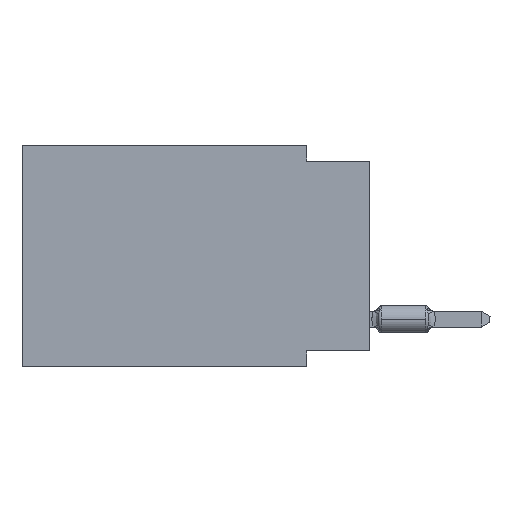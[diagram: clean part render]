
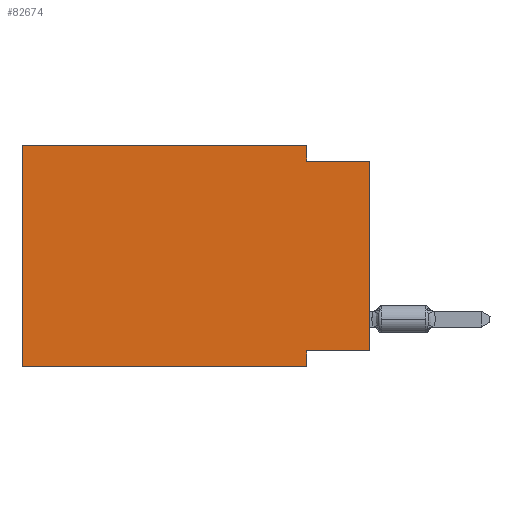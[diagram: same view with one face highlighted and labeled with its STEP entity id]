
A CAD part, left-side view. The second image highlights one B-rep face of the part: STEP entity #82674.
In plain terms, the highlighted planar face has unit normal (-1, 0, 0).
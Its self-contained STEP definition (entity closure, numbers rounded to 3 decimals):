
#1590 = CARTESIAN_POINT ( 'NONE',  ( 0., 0., 0. ) ) ;
#4566 = VECTOR ( 'NONE', #47866, 1000. ) ;
#7027 = VECTOR ( 'NONE', #30321, 1000. ) ;
#7937 = CARTESIAN_POINT ( 'NONE',  ( 0., 13.97, 0. ) ) ;
#10151 = VECTOR ( 'NONE', #42380, 1000. ) ;
#12165 = VERTEX_POINT ( 'NONE', #28537 ) ;
#12567 = ORIENTED_EDGE ( 'NONE', *, *, #30296, .F. ) ;
#13518 = CARTESIAN_POINT ( 'NONE',  ( 0., 0., -8.255 ) ) ;
#17027 = LINE ( 'NONE', #49038, #84397 ) ;
#19657 = ORIENTED_EDGE ( 'NONE', *, *, #29262, .T. ) ;
#20158 = ORIENTED_EDGE ( 'NONE', *, *, #67251, .F. ) ;
#21334 = LINE ( 'NONE', #104791, #4566 ) ;
#22619 = DIRECTION ( 'NONE',  ( 0., 0., -1. ) ) ;
#24917 = LINE ( 'NONE', #1590, #84020 ) ;
#27387 = VECTOR ( 'NONE', #83274, 1000. ) ;
#28537 = CARTESIAN_POINT ( 'NONE',  ( 0., 2.54, -8.255 ) ) ;
#29262 = EDGE_CURVE ( 'NONE', #103199, #61227, #24917, .T. ) ;
#29929 = EDGE_CURVE ( 'NONE', #106783, #54262, #37725, .T. ) ;
#30296 = EDGE_CURVE ( 'NONE', #78901, #106783, #21334, .T. ) ;
#30321 = DIRECTION ( 'NONE',  ( 0., 1., 0. ) ) ;
#30520 = VERTEX_POINT ( 'NONE', #58142 ) ;
#30572 = CARTESIAN_POINT ( 'NONE',  ( 0., 13.97, 0. ) ) ;
#37725 = LINE ( 'NONE', #47454, #77249 ) ;
#38580 = AXIS2_PLACEMENT_3D ( 'NONE', #7937, #41013, #107128 ) ;
#38893 = LINE ( 'NONE', #48086, #71156 ) ;
#41013 = DIRECTION ( 'NONE',  ( 1., 0., 0. ) ) ;
#42380 = DIRECTION ( 'NONE',  ( 0., 0., -1. ) ) ;
#43558 = CARTESIAN_POINT ( 'NONE',  ( 0., 0., -0.635 ) ) ;
#46157 = ORIENTED_EDGE ( 'NONE', *, *, #65467, .F. ) ;
#46652 = CARTESIAN_POINT ( 'NONE',  ( 0., 13.97, -8.89 ) ) ;
#47454 = CARTESIAN_POINT ( 'NONE',  ( 0., 13.97, 0. ) ) ;
#47866 = DIRECTION ( 'NONE',  ( 0., 0., 1. ) ) ;
#48086 = CARTESIAN_POINT ( 'NONE',  ( 0., 2.54, 0. ) ) ;
#48791 = EDGE_LOOP ( 'NONE', ( #19657, #105285, #20158, #94093, #12567, #75401, #87967, #46157 ) ) ;
#49038 = CARTESIAN_POINT ( 'NONE',  ( 0., 13.97, -8.89 ) ) ;
#49152 = PLANE ( 'NONE',  #38580 ) ;
#50525 = LINE ( 'NONE', #59735, #10151 ) ;
#54262 = VERTEX_POINT ( 'NONE', #60885 ) ;
#54734 = LINE ( 'NONE', #13518, #7027 ) ;
#58142 = CARTESIAN_POINT ( 'NONE',  ( 0., 2.54, -0.635 ) ) ;
#59735 = CARTESIAN_POINT ( 'NONE',  ( 0., 2.54, -8.89 ) ) ;
#60359 = EDGE_CURVE ( 'NONE', #12165, #64620, #50525, .T. ) ;
#60885 = CARTESIAN_POINT ( 'NONE',  ( 0., 2.54, 0. ) ) ;
#61227 = VERTEX_POINT ( 'NONE', #43558 ) ;
#63207 = DIRECTION ( 'NONE',  ( 0., -1., 0. ) ) ;
#64620 = VERTEX_POINT ( 'NONE', #78318 ) ;
#65467 = EDGE_CURVE ( 'NONE', #103199, #12165, #54734, .T. ) ;
#67251 = EDGE_CURVE ( 'NONE', #54262, #30520, #38893, .T. ) ;
#71156 = VECTOR ( 'NONE', #22619, 1000. ) ;
#75401 = ORIENTED_EDGE ( 'NONE', *, *, #75894, .T. ) ;
#75894 = EDGE_CURVE ( 'NONE', #78901, #64620, #17027, .T. ) ;
#76543 = EDGE_CURVE ( 'NONE', #30520, #61227, #106073, .T. ) ;
#77249 = VECTOR ( 'NONE', #63207, 1000. ) ;
#78318 = CARTESIAN_POINT ( 'NONE',  ( 0., 2.54, -8.89 ) ) ;
#78901 = VERTEX_POINT ( 'NONE', #46652 ) ;
#81551 = DIRECTION ( 'NONE',  ( 0., -1., 0. ) ) ;
#82674 = ADVANCED_FACE ( 'NONE', ( #90335 ), #49152, .F. ) ;
#83274 = DIRECTION ( 'NONE',  ( 0., -1., 0. ) ) ;
#84020 = VECTOR ( 'NONE', #91567, 1000. ) ;
#84397 = VECTOR ( 'NONE', #81551, 1000. ) ;
#87967 = ORIENTED_EDGE ( 'NONE', *, *, #60359, .F. ) ;
#90335 = FACE_OUTER_BOUND ( 'NONE', #48791, .T. ) ;
#91567 = DIRECTION ( 'NONE',  ( 0., 0., 1. ) ) ;
#94093 = ORIENTED_EDGE ( 'NONE', *, *, #29929, .F. ) ;
#97404 = CARTESIAN_POINT ( 'NONE',  ( 0., 0., -0.635 ) ) ;
#100927 = CARTESIAN_POINT ( 'NONE',  ( 0., 0., -8.255 ) ) ;
#103199 = VERTEX_POINT ( 'NONE', #100927 ) ;
#104791 = CARTESIAN_POINT ( 'NONE',  ( 0., 13.97, 0. ) ) ;
#105285 = ORIENTED_EDGE ( 'NONE', *, *, #76543, .F. ) ;
#106073 = LINE ( 'NONE', #97404, #27387 ) ;
#106783 = VERTEX_POINT ( 'NONE', #30572 ) ;
#107128 = DIRECTION ( 'NONE',  ( 0., 0., -1. ) ) ;
